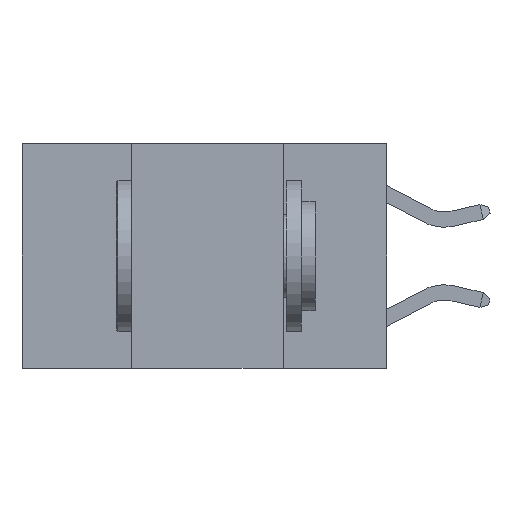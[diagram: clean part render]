
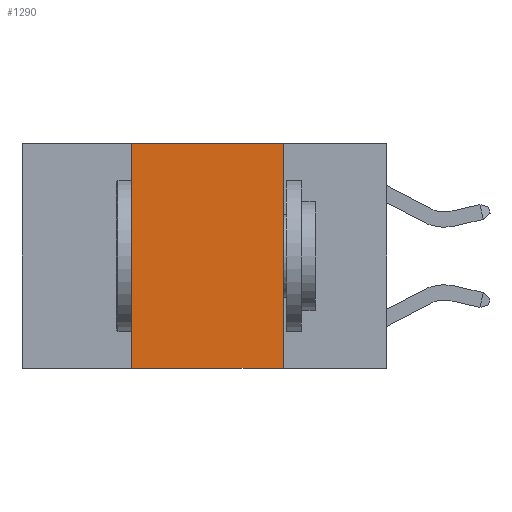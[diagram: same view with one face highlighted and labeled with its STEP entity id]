
A CAD part, left-side view. The second image highlights one B-rep face of the part: STEP entity #1290.
In plain terms, the highlighted planar face has unit normal (-1, 0, 0).
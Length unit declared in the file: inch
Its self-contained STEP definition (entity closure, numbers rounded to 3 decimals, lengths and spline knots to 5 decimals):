
#374 = CARTESIAN_POINT ( 'NONE',  ( 0., 0.6, -0.37 ) ) ;
#1290 = ADVANCED_FACE ( 'NONE', ( #3086 ), #1874, .F. ) ;
#1684 = DIRECTION ( 'NONE',  ( 0., 0., -1. ) ) ;
#1706 = DIRECTION ( 'NONE',  ( 1., 0., 0. ) ) ;
#1755 = CARTESIAN_POINT ( 'NONE',  ( 0., 0.6, 0. ) ) ;
#1874 = PLANE ( 'NONE',  #10595 ) ;
#2208 = LINE ( 'NONE', #11549, #12540 ) ;
#2505 = CARTESIAN_POINT ( 'NONE',  ( 0., 0.17, 0. ) ) ;
#2739 = DIRECTION ( 'NONE',  ( 0., -1., 0. ) ) ;
#2948 = VERTEX_POINT ( 'NONE', #15252 ) ;
#3086 = FACE_OUTER_BOUND ( 'NONE', #12614, .T. ) ;
#3827 = ORIENTED_EDGE ( 'NONE', *, *, #5138, .F. ) ;
#4066 = LINE ( 'NONE', #374, #6781 ) ;
#4170 = CARTESIAN_POINT ( 'NONE',  ( 0., 0.17, -0.37 ) ) ;
#4350 = CARTESIAN_POINT ( 'NONE',  ( 0., 0.17, 0. ) ) ;
#4505 = VERTEX_POINT ( 'NONE', #4170 ) ;
#5138 = EDGE_CURVE ( 'NONE', #15670, #15754, #16213, .T. ) ;
#6036 = VECTOR ( 'NONE', #2739, 39.37008 ) ;
#6781 = VECTOR ( 'NONE', #9973, 39.37008 ) ;
#7969 = EDGE_CURVE ( 'NONE', #2948, #4505, #4066, .T. ) ;
#9091 = EDGE_CURVE ( 'NONE', #15754, #4505, #16957, .T. ) ;
#9470 = CARTESIAN_POINT ( 'NONE',  ( 0., 0.6, 0. ) ) ;
#9751 = EDGE_CURVE ( 'NONE', #2948, #15670, #2208, .T. ) ;
#9973 = DIRECTION ( 'NONE',  ( 0., -1., 0. ) ) ;
#10083 = ORIENTED_EDGE ( 'NONE', *, *, #9091, .F. ) ;
#10225 = DIRECTION ( 'NONE',  ( 0., 0., 1. ) ) ;
#10595 = AXIS2_PLACEMENT_3D ( 'NONE', #1755, #1706, #1684 ) ;
#10925 = ORIENTED_EDGE ( 'NONE', *, *, #9751, .F. ) ;
#11333 = ORIENTED_EDGE ( 'NONE', *, *, #7969, .T. ) ;
#11549 = CARTESIAN_POINT ( 'NONE',  ( 0., 0.42, 0. ) ) ;
#12540 = VECTOR ( 'NONE', #10225, 39.37008 ) ;
#12614 = EDGE_LOOP ( 'NONE', ( #10083, #3827, #10925, #11333 ) ) ;
#13377 = VECTOR ( 'NONE', #15957, 39.37008 ) ;
#13398 = CARTESIAN_POINT ( 'NONE',  ( 0., 0.42, 0. ) ) ;
#15252 = CARTESIAN_POINT ( 'NONE',  ( 0., 0.42, -0.37 ) ) ;
#15670 = VERTEX_POINT ( 'NONE', #13398 ) ;
#15754 = VERTEX_POINT ( 'NONE', #4350 ) ;
#15957 = DIRECTION ( 'NONE',  ( 0., 0., -1. ) ) ;
#16213 = LINE ( 'NONE', #9470, #6036 ) ;
#16957 = LINE ( 'NONE', #2505, #13377 ) ;
